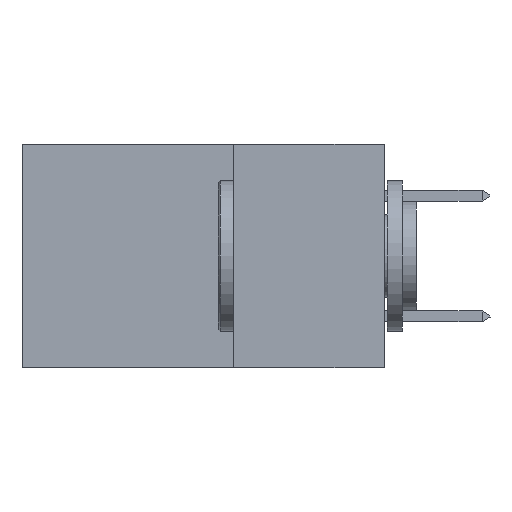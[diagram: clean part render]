
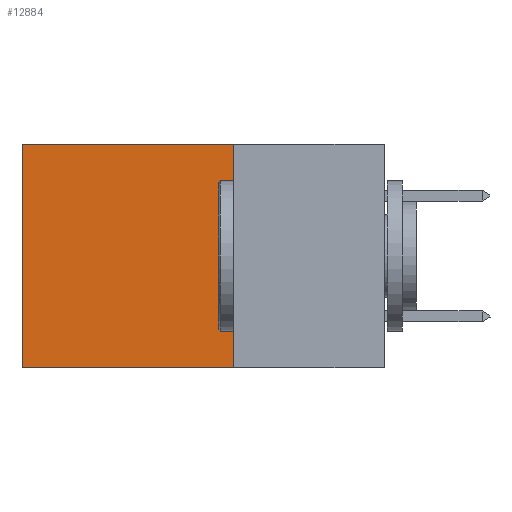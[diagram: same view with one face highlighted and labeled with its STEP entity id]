
A CAD part, left-side view. The second image highlights one B-rep face of the part: STEP entity #12884.
In plain terms, the highlighted planar face has unit normal (-1, 0, 0).
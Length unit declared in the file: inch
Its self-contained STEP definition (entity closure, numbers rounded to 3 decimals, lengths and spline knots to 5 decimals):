
#65 = CARTESIAN_POINT ( 'NONE',  ( 0.2875, 0.6, -0.37 ) ) ;
#461 = DIRECTION ( 'NONE',  ( 0., 0., -1. ) ) ;
#1142 = VERTEX_POINT ( 'NONE', #65 ) ;
#1326 = DIRECTION ( 'NONE',  ( 1., 0., 0. ) ) ;
#1589 = VERTEX_POINT ( 'NONE', #5037 ) ;
#2683 = DIRECTION ( 'NONE',  ( 0., 0., -1. ) ) ;
#3311 = DIRECTION ( 'NONE',  ( 0., 1., 0. ) ) ;
#4313 = VERTEX_POINT ( 'NONE', #7911 ) ;
#4366 = ORIENTED_EDGE ( 'NONE', *, *, #16000, .T. ) ;
#5037 = CARTESIAN_POINT ( 'NONE',  ( 0.2875, 0.25, -0.37 ) ) ;
#7542 = ORIENTED_EDGE ( 'NONE', *, *, #12981, .T. ) ;
#7886 = AXIS2_PLACEMENT_3D ( 'NONE', #11063, #1326, #12605 ) ;
#7897 = PLANE ( 'NONE',  #7886 ) ;
#7911 = CARTESIAN_POINT ( 'NONE',  ( 0.2875, 0.6, 0. ) ) ;
#8013 = ORIENTED_EDGE ( 'NONE', *, *, #10365, .F. ) ;
#8943 = LINE ( 'NONE', #13740, #16515 ) ;
#9771 = EDGE_LOOP ( 'NONE', ( #4366, #9958, #8013, #7542 ) ) ;
#9958 = ORIENTED_EDGE ( 'NONE', *, *, #17231, .F. ) ;
#10365 = EDGE_CURVE ( 'NONE', #18920, #1589, #8943, .T. ) ;
#10405 = LINE ( 'NONE', #13280, #17394 ) ;
#11063 = CARTESIAN_POINT ( 'NONE',  ( 0.2875, 0.25, 0. ) ) ;
#11969 = DIRECTION ( 'NONE',  ( 0., 1., 0. ) ) ;
#12605 = DIRECTION ( 'NONE',  ( 0., 0., -1. ) ) ;
#12884 = ADVANCED_FACE ( 'NONE', ( #16645 ), #7897, .F. ) ;
#12981 = EDGE_CURVE ( 'NONE', #18920, #4313, #15276, .T. ) ;
#13280 = CARTESIAN_POINT ( 'NONE',  ( 0.2875, 0.6, 0. ) ) ;
#13740 = CARTESIAN_POINT ( 'NONE',  ( 0.2875, 0.25, 0. ) ) ;
#15276 = LINE ( 'NONE', #19985, #18213 ) ;
#15317 = LINE ( 'NONE', #16398, #17798 ) ;
#16000 = EDGE_CURVE ( 'NONE', #4313, #1142, #10405, .T. ) ;
#16398 = CARTESIAN_POINT ( 'NONE',  ( 0.2875, 0.25, -0.37 ) ) ;
#16496 = CARTESIAN_POINT ( 'NONE',  ( 0.2875, 0.25, 0. ) ) ;
#16515 = VECTOR ( 'NONE', #2683, 39.37008 ) ;
#16645 = FACE_OUTER_BOUND ( 'NONE', #9771, .T. ) ;
#17231 = EDGE_CURVE ( 'NONE', #1589, #1142, #15317, .T. ) ;
#17394 = VECTOR ( 'NONE', #461, 39.37008 ) ;
#17798 = VECTOR ( 'NONE', #11969, 39.37008 ) ;
#18213 = VECTOR ( 'NONE', #3311, 39.37008 ) ;
#18920 = VERTEX_POINT ( 'NONE', #16496 ) ;
#19985 = CARTESIAN_POINT ( 'NONE',  ( 0.2875, 0.25, 0. ) ) ;
